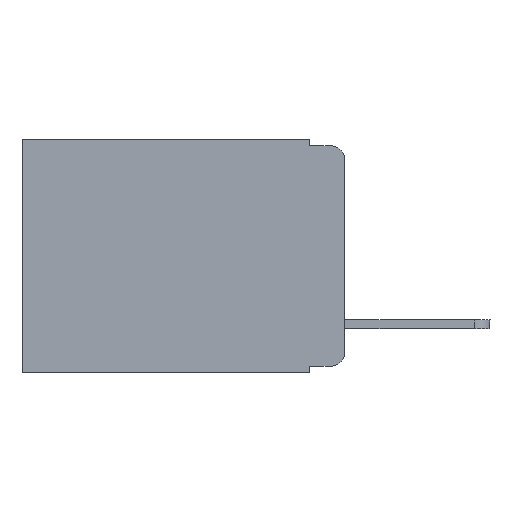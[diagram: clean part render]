
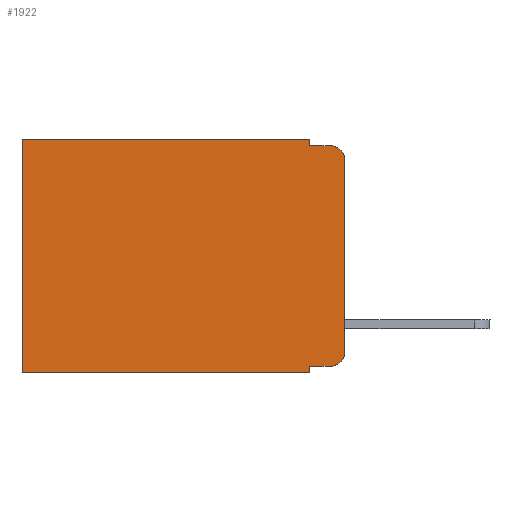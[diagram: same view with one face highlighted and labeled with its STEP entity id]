
A CAD part, left-side view. The second image highlights one B-rep face of the part: STEP entity #1922.
In plain terms, the highlighted planar face has unit normal (-1, 0, 0).
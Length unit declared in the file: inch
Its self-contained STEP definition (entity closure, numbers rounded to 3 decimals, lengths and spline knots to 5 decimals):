
#116 = VECTOR ( 'NONE', #18132, 39.37008 ) ;
#260 = CARTESIAN_POINT ( 'NONE',  ( 0.298, 0.473, 0. ) ) ;
#329 = DIRECTION ( 'NONE',  ( 0., 0., -1. ) ) ;
#616 = CARTESIAN_POINT ( 'NONE',  ( 0.298, 0.051, -0.01 ) ) ;
#738 = CARTESIAN_POINT ( 'NONE',  ( 0.298, 0., 0. ) ) ;
#798 = LINE ( 'NONE', #10367, #13393 ) ;
#802 = CARTESIAN_POINT ( 'NONE',  ( 0.298, 0.051, -0.343 ) ) ;
#831 = ORIENTED_EDGE ( 'NONE', *, *, #18264, .F. ) ;
#838 = ORIENTED_EDGE ( 'NONE', *, *, #1082, .T. ) ;
#891 = ORIENTED_EDGE ( 'NONE', *, *, #15259, .T. ) ;
#928 = CARTESIAN_POINT ( 'NONE',  ( 0.298, 0.02, -0.333 ) ) ;
#1056 = ORIENTED_EDGE ( 'NONE', *, *, #2816, .F. ) ;
#1082 = EDGE_CURVE ( 'NONE', #2658, #15344, #17822, .T. ) ;
#1138 = EDGE_CURVE ( 'NONE', #19630, #11623, #13469, .T. ) ;
#1418 = VERTEX_POINT ( 'NONE', #17287 ) ;
#1568 = CARTESIAN_POINT ( 'NONE',  ( 0.298, 0.473, -0.343 ) ) ;
#1922 = ADVANCED_FACE ( 'NONE', ( #10009 ), #19465, .F. ) ;
#1955 = VECTOR ( 'NONE', #2369, 39.37008 ) ;
#2008 = CARTESIAN_POINT ( 'NONE',  ( 0.298, 0.051, -0.333 ) ) ;
#2171 = DIRECTION ( 'NONE',  ( 0., 0., -1. ) ) ;
#2369 = DIRECTION ( 'NONE',  ( 0., 0., -1. ) ) ;
#2658 = VERTEX_POINT ( 'NONE', #928 ) ;
#2816 = EDGE_CURVE ( 'NONE', #9921, #19630, #20228, .T. ) ;
#3119 = ORIENTED_EDGE ( 'NONE', *, *, #17990, .F. ) ;
#3776 = VERTEX_POINT ( 'NONE', #15408 ) ;
#3899 = DIRECTION ( 'NONE',  ( 0., 0., -1. ) ) ;
#3980 = CARTESIAN_POINT ( 'NONE',  ( 0.298, 0.051, 0. ) ) ;
#4279 = AXIS2_PLACEMENT_3D ( 'NONE', #13101, #17764, #14811 ) ;
#4738 = LINE ( 'NONE', #10803, #20856 ) ;
#5031 = DIRECTION ( 'NONE',  ( 1., 0., 0. ) ) ;
#5948 = VECTOR ( 'NONE', #9855, 39.37008 ) ;
#6267 = ORIENTED_EDGE ( 'NONE', *, *, #1138, .F. ) ;
#6987 = VECTOR ( 'NONE', #16915, 39.37008 ) ;
#8271 = EDGE_CURVE ( 'NONE', #3776, #11790, #11067, .T. ) ;
#8449 = EDGE_CURVE ( 'NONE', #13961, #1418, #15228, .T. ) ;
#8885 = CARTESIAN_POINT ( 'NONE',  ( 0.298, 0.02, -0.01 ) ) ;
#9855 = DIRECTION ( 'NONE',  ( 0., 1., 0. ) ) ;
#9921 = VERTEX_POINT ( 'NONE', #2008 ) ;
#9957 = CARTESIAN_POINT ( 'NONE',  ( 0.298, 0.051, 0. ) ) ;
#10009 = FACE_OUTER_BOUND ( 'NONE', #18138, .T. ) ;
#10058 = DIRECTION ( 'NONE',  ( -1., 0., 0. ) ) ;
#10367 = CARTESIAN_POINT ( 'NONE',  ( 0.298, 0., 0. ) ) ;
#10803 = CARTESIAN_POINT ( 'NONE',  ( 0.298, 0.051, -0.333 ) ) ;
#10888 = ORIENTED_EDGE ( 'NONE', *, *, #19805, .T. ) ;
#11067 = CIRCLE ( 'NONE', #4279, 0.02 ) ;
#11623 = VERTEX_POINT ( 'NONE', #1568 ) ;
#11661 = DIRECTION ( 'NONE',  ( 0., 0., -1. ) ) ;
#11790 = VERTEX_POINT ( 'NONE', #8885 ) ;
#12398 = AXIS2_PLACEMENT_3D ( 'NONE', #13160, #10058, #11661 ) ;
#13101 = CARTESIAN_POINT ( 'NONE',  ( 0.298, 0.02, -0.03 ) ) ;
#13160 = CARTESIAN_POINT ( 'NONE',  ( 0.298, 0.02, -0.313 ) ) ;
#13393 = VECTOR ( 'NONE', #3899, 39.37008 ) ;
#13469 = LINE ( 'NONE', #19728, #5948 ) ;
#13598 = DIRECTION ( 'NONE',  ( 0., -1., 0. ) ) ;
#13615 = AXIS2_PLACEMENT_3D ( 'NONE', #14709, #5031, #329 ) ;
#13644 = VERTEX_POINT ( 'NONE', #16970 ) ;
#13961 = VERTEX_POINT ( 'NONE', #16534 ) ;
#14304 = VECTOR ( 'NONE', #2171, 39.37008 ) ;
#14709 = CARTESIAN_POINT ( 'NONE',  ( 0.298, 0., 0. ) ) ;
#14811 = DIRECTION ( 'NONE',  ( 0., 0., -1. ) ) ;
#15209 = LINE ( 'NONE', #616, #20837 ) ;
#15228 = LINE ( 'NONE', #738, #6987 ) ;
#15259 = EDGE_CURVE ( 'NONE', #1418, #11623, #16746, .T. ) ;
#15344 = VERTEX_POINT ( 'NONE', #18109 ) ;
#15408 = CARTESIAN_POINT ( 'NONE',  ( 0.298, 0., -0.03 ) ) ;
#15948 = ORIENTED_EDGE ( 'NONE', *, *, #18403, .F. ) ;
#16534 = CARTESIAN_POINT ( 'NONE',  ( 0.298, 0.051, 0. ) ) ;
#16746 = LINE ( 'NONE', #260, #14304 ) ;
#16915 = DIRECTION ( 'NONE',  ( 0., 1., 0. ) ) ;
#16970 = CARTESIAN_POINT ( 'NONE',  ( 0.298, 0.051, -0.01 ) ) ;
#17287 = CARTESIAN_POINT ( 'NONE',  ( 0.298, 0.473, 0. ) ) ;
#17294 = DIRECTION ( 'NONE',  ( 0., -1., 0. ) ) ;
#17764 = DIRECTION ( 'NONE',  ( -1., 0., 0. ) ) ;
#17822 = CIRCLE ( 'NONE', #12398, 0.02 ) ;
#17990 = EDGE_CURVE ( 'NONE', #13644, #11790, #15209, .T. ) ;
#18094 = ORIENTED_EDGE ( 'NONE', *, *, #8271, .T. ) ;
#18109 = CARTESIAN_POINT ( 'NONE',  ( 0.298, 0., -0.313 ) ) ;
#18132 = DIRECTION ( 'NONE',  ( 0., 0., -1. ) ) ;
#18138 = EDGE_LOOP ( 'NONE', ( #15948, #18094, #3119, #831, #19471, #891, #6267, #1056, #10888, #838 ) ) ;
#18264 = EDGE_CURVE ( 'NONE', #13961, #13644, #19732, .T. ) ;
#18403 = EDGE_CURVE ( 'NONE', #3776, #15344, #798, .T. ) ;
#19465 = PLANE ( 'NONE',  #13615 ) ;
#19471 = ORIENTED_EDGE ( 'NONE', *, *, #8449, .T. ) ;
#19630 = VERTEX_POINT ( 'NONE', #802 ) ;
#19728 = CARTESIAN_POINT ( 'NONE',  ( 0.298, 0., -0.343 ) ) ;
#19732 = LINE ( 'NONE', #9957, #116 ) ;
#19805 = EDGE_CURVE ( 'NONE', #9921, #2658, #4738, .T. ) ;
#20228 = LINE ( 'NONE', #3980, #1955 ) ;
#20837 = VECTOR ( 'NONE', #13598, 39.37008 ) ;
#20856 = VECTOR ( 'NONE', #17294, 39.37008 ) ;
